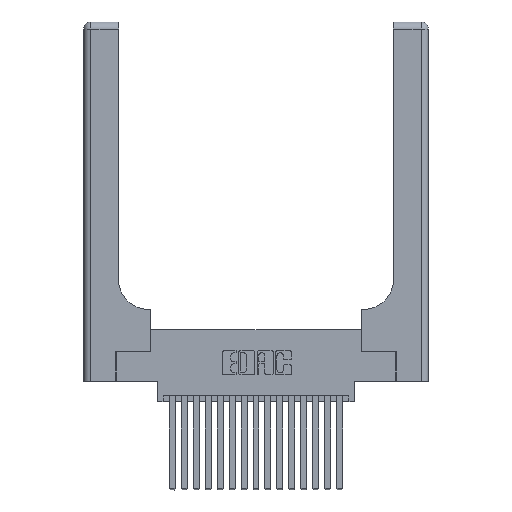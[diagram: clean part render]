
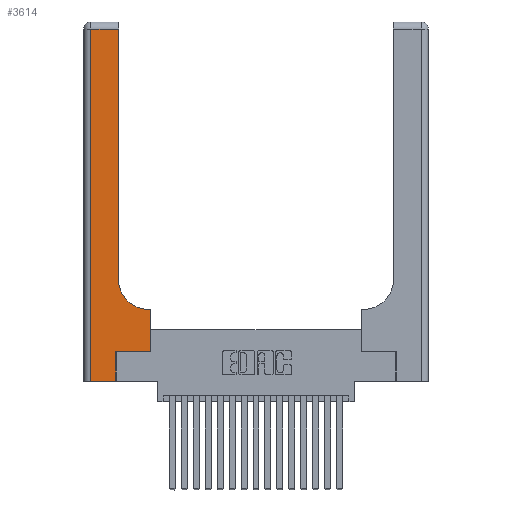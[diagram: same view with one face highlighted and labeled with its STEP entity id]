
A CAD part, top view. The second image highlights one B-rep face of the part: STEP entity #3614.
In plain terms, the highlighted planar face has unit normal (0, 0, 1).
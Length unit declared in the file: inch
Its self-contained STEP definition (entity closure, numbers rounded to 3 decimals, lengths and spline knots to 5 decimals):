
#11 = CARTESIAN_POINT ( 'NONE',  ( 0.5585, 0.25, 0.37 ) ) ;
#499 = LINE ( 'NONE', #9011, #6679 ) ;
#587 = VECTOR ( 'NONE', #9343, 39.37008 ) ;
#619 = LINE ( 'NONE', #4675, #868 ) ;
#677 = CARTESIAN_POINT ( 'NONE',  ( 0.5415, 0.85, 0.37 ) ) ;
#868 = VECTOR ( 'NONE', #6237, 39.37008 ) ;
#1241 = CARTESIAN_POINT ( 'NONE',  ( 0.06, 2.94, 0.37 ) ) ;
#1543 = CARTESIAN_POINT ( 'NONE',  ( 0., 0., 0.37 ) ) ;
#2049 = EDGE_CURVE ( 'NONE', #18374, #18426, #9645, .T. ) ;
#2258 = ORIENTED_EDGE ( 'NONE', *, *, #17218, .T. ) ;
#2465 = VERTEX_POINT ( 'NONE', #10273 ) ;
#2655 = LINE ( 'NONE', #6389, #13840 ) ;
#2659 = VECTOR ( 'NONE', #12670, 39.37008 ) ;
#2992 = CARTESIAN_POINT ( 'NONE',  ( 0.269, 0., 0.37 ) ) ;
#3035 = DIRECTION ( 'NONE',  ( 0., 1., 0. ) ) ;
#3224 = DIRECTION ( 'NONE',  ( 0., 1., 0. ) ) ;
#3569 = AXIS2_PLACEMENT_3D ( 'NONE', #10084, #17888, #5346 ) ;
#3614 = ADVANCED_FACE ( 'NONE', ( #10330 ), #18030, .F. ) ;
#4220 = VERTEX_POINT ( 'NONE', #11 ) ;
#4364 = LINE ( 'NONE', #16287, #9586 ) ;
#4675 = CARTESIAN_POINT ( 'NONE',  ( 0.269, 0., 0.37 ) ) ;
#4866 = EDGE_CURVE ( 'NONE', #8646, #18677, #18217, .T. ) ;
#5170 = ORIENTED_EDGE ( 'NONE', *, *, #14551, .T. ) ;
#5346 = DIRECTION ( 'NONE',  ( -1., 0., 0. ) ) ;
#5435 = CARTESIAN_POINT ( 'NONE',  ( 0.06, 0., 0.37 ) ) ;
#5529 = ORIENTED_EDGE ( 'NONE', *, *, #2049, .T. ) ;
#5741 = VECTOR ( 'NONE', #13700, 39.37008 ) ;
#6237 = DIRECTION ( 'NONE',  ( 0., 1., 0. ) ) ;
#6268 = CARTESIAN_POINT ( 'NONE',  ( 0.2915, 3., 0.37 ) ) ;
#6389 = CARTESIAN_POINT ( 'NONE',  ( 0.5585, 0.25, 0.37 ) ) ;
#6679 = VECTOR ( 'NONE', #20138, 39.37008 ) ;
#6744 = LINE ( 'NONE', #8836, #5741 ) ;
#6906 = ORIENTED_EDGE ( 'NONE', *, *, #9341, .T. ) ;
#7363 = EDGE_LOOP ( 'NONE', ( #5170, #7433, #10372, #2258, #14454, #6906, #15280, #15025, #5529 ) ) ;
#7433 = ORIENTED_EDGE ( 'NONE', *, *, #12859, .T. ) ;
#8618 = LINE ( 'NONE', #1543, #2659 ) ;
#8646 = VERTEX_POINT ( 'NONE', #1241 ) ;
#8836 = CARTESIAN_POINT ( 'NONE',  ( 0., 2.94, 0.37 ) ) ;
#9011 = CARTESIAN_POINT ( 'NONE',  ( 0.2915, 0.6, 0.37 ) ) ;
#9341 = EDGE_CURVE ( 'NONE', #10851, #4220, #4364, .T. ) ;
#9343 = DIRECTION ( 'NONE',  ( 0., -1., 0. ) ) ;
#9374 = CARTESIAN_POINT ( 'NONE',  ( 0.5415, 0.6, 0.37 ) ) ;
#9586 = VECTOR ( 'NONE', #19313, 39.37008 ) ;
#9645 = CIRCLE ( 'NONE', #13575, 0.25 ) ;
#10084 = CARTESIAN_POINT ( 'NONE',  ( 0., 3., 0.37 ) ) ;
#10273 = CARTESIAN_POINT ( 'NONE',  ( 0.2915, 2.94, 0.37 ) ) ;
#10330 = FACE_OUTER_BOUND ( 'NONE', #7363, .T. ) ;
#10372 = ORIENTED_EDGE ( 'NONE', *, *, #4866, .T. ) ;
#10851 = VERTEX_POINT ( 'NONE', #17838 ) ;
#10950 = VECTOR ( 'NONE', #3035, 39.37008 ) ;
#11460 = CARTESIAN_POINT ( 'NONE',  ( 0.2915, 0.85, 0.37 ) ) ;
#11937 = DIRECTION ( 'NONE',  ( 0., 0., -1. ) ) ;
#12070 = EDGE_CURVE ( 'NONE', #20128, #10851, #619, .T. ) ;
#12481 = CARTESIAN_POINT ( 'NONE',  ( 0.06, 3., 0.37 ) ) ;
#12670 = DIRECTION ( 'NONE',  ( 1., 0., 0. ) ) ;
#12859 = EDGE_CURVE ( 'NONE', #2465, #8646, #6744, .T. ) ;
#13575 = AXIS2_PLACEMENT_3D ( 'NONE', #677, #11937, #19793 ) ;
#13700 = DIRECTION ( 'NONE',  ( -1., 0., 0. ) ) ;
#13840 = VECTOR ( 'NONE', #3224, 39.37008 ) ;
#14454 = ORIENTED_EDGE ( 'NONE', *, *, #12070, .T. ) ;
#14551 = EDGE_CURVE ( 'NONE', #18426, #2465, #17181, .T. ) ;
#14740 = VERTEX_POINT ( 'NONE', #17545 ) ;
#15025 = ORIENTED_EDGE ( 'NONE', *, *, #18805, .T. ) ;
#15280 = ORIENTED_EDGE ( 'NONE', *, *, #16581, .T. ) ;
#16287 = CARTESIAN_POINT ( 'NONE',  ( 0.269, 0.25, 0.37 ) ) ;
#16581 = EDGE_CURVE ( 'NONE', #4220, #14740, #2655, .T. ) ;
#17181 = LINE ( 'NONE', #6268, #10950 ) ;
#17218 = EDGE_CURVE ( 'NONE', #18677, #20128, #8618, .T. ) ;
#17545 = CARTESIAN_POINT ( 'NONE',  ( 0.5585, 0.6, 0.37 ) ) ;
#17838 = CARTESIAN_POINT ( 'NONE',  ( 0.269, 0.25, 0.37 ) ) ;
#17888 = DIRECTION ( 'NONE',  ( 0., 0., -1. ) ) ;
#18030 = PLANE ( 'NONE',  #3569 ) ;
#18217 = LINE ( 'NONE', #12481, #587 ) ;
#18374 = VERTEX_POINT ( 'NONE', #9374 ) ;
#18426 = VERTEX_POINT ( 'NONE', #11460 ) ;
#18677 = VERTEX_POINT ( 'NONE', #5435 ) ;
#18805 = EDGE_CURVE ( 'NONE', #14740, #18374, #499, .T. ) ;
#19313 = DIRECTION ( 'NONE',  ( 1., 0., 0. ) ) ;
#19793 = DIRECTION ( 'NONE',  ( 1., 0., 0. ) ) ;
#20128 = VERTEX_POINT ( 'NONE', #2992 ) ;
#20138 = DIRECTION ( 'NONE',  ( -1., 0., 0. ) ) ;
